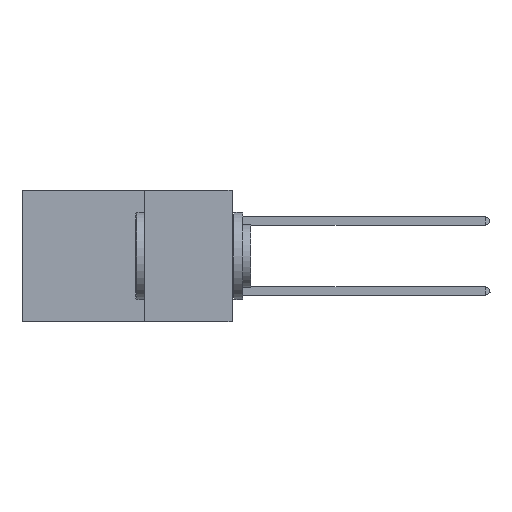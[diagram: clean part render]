
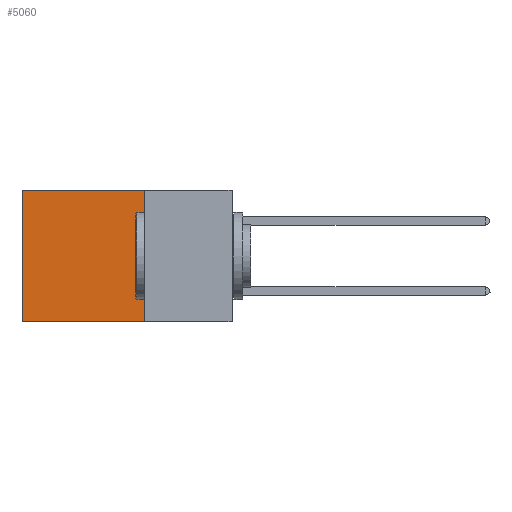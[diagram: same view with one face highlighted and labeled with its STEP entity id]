
A CAD part, left-side view. The second image highlights one B-rep face of the part: STEP entity #5060.
In plain terms, the highlighted planar face has unit normal (-1, 0, 0).
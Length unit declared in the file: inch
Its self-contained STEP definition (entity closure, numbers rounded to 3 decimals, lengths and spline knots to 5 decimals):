
#556 = CARTESIAN_POINT ( 'NONE',  ( 0.2875, 0.6, -0.375 ) ) ;
#1638 = DIRECTION ( 'NONE',  ( 0., 0., -1. ) ) ;
#2594 = PLANE ( 'NONE',  #7044 ) ;
#2884 = ORIENTED_EDGE ( 'NONE', *, *, #15288, .F. ) ;
#3724 = VERTEX_POINT ( 'NONE', #5631 ) ;
#5060 = ADVANCED_FACE ( 'NONE', ( #6014 ), #2594, .F. ) ;
#5631 = CARTESIAN_POINT ( 'NONE',  ( 0.2875, 0.25, -0.375 ) ) ;
#5751 = EDGE_CURVE ( 'NONE', #3724, #15061, #11665, .T. ) ;
#6014 = FACE_OUTER_BOUND ( 'NONE', #13826, .T. ) ;
#6790 = VECTOR ( 'NONE', #1638, 39.37008 ) ;
#7044 = AXIS2_PLACEMENT_3D ( 'NONE', #21666, #16665, #7859 ) ;
#7726 = CARTESIAN_POINT ( 'NONE',  ( 0.2875, 0.6, -0.375 ) ) ;
#7859 = DIRECTION ( 'NONE',  ( 0., 0., -1. ) ) ;
#7954 = DIRECTION ( 'NONE',  ( 0., 1., 0. ) ) ;
#8701 = VECTOR ( 'NONE', #21928, 39.37008 ) ;
#9103 = EDGE_CURVE ( 'NONE', #15189, #21545, #17268, .T. ) ;
#9118 = DIRECTION ( 'NONE',  ( 0., 0., -1. ) ) ;
#9856 = CARTESIAN_POINT ( 'NONE',  ( 0.2875, 0.25, -0.375 ) ) ;
#10861 = LINE ( 'NONE', #18911, #6790 ) ;
#11665 = LINE ( 'NONE', #9856, #8701 ) ;
#12656 = VECTOR ( 'NONE', #7954, 39.37008 ) ;
#12912 = ORIENTED_EDGE ( 'NONE', *, *, #5751, .F. ) ;
#13388 = CARTESIAN_POINT ( 'NONE',  ( 0.2875, 0.25, 0. ) ) ;
#13826 = EDGE_LOOP ( 'NONE', ( #15127, #12912, #2884, #15007 ) ) ;
#14253 = VECTOR ( 'NONE', #9118, 39.37008 ) ;
#15007 = ORIENTED_EDGE ( 'NONE', *, *, #9103, .T. ) ;
#15061 = VERTEX_POINT ( 'NONE', #7726 ) ;
#15127 = ORIENTED_EDGE ( 'NONE', *, *, #18110, .T. ) ;
#15189 = VERTEX_POINT ( 'NONE', #13388 ) ;
#15288 = EDGE_CURVE ( 'NONE', #15189, #3724, #10861, .T. ) ;
#15661 = CARTESIAN_POINT ( 'NONE',  ( 0.2875, 0.6, 0. ) ) ;
#16536 = CARTESIAN_POINT ( 'NONE',  ( 0.2875, 0.25, 0. ) ) ;
#16665 = DIRECTION ( 'NONE',  ( 1., 0., 0. ) ) ;
#17197 = LINE ( 'NONE', #556, #14253 ) ;
#17268 = LINE ( 'NONE', #16536, #12656 ) ;
#18110 = EDGE_CURVE ( 'NONE', #21545, #15061, #17197, .T. ) ;
#18911 = CARTESIAN_POINT ( 'NONE',  ( 0.2875, 0.25, -0.375 ) ) ;
#21545 = VERTEX_POINT ( 'NONE', #15661 ) ;
#21666 = CARTESIAN_POINT ( 'NONE',  ( 0.2875, 0.25, -0.375 ) ) ;
#21928 = DIRECTION ( 'NONE',  ( 0., 1., 0. ) ) ;
